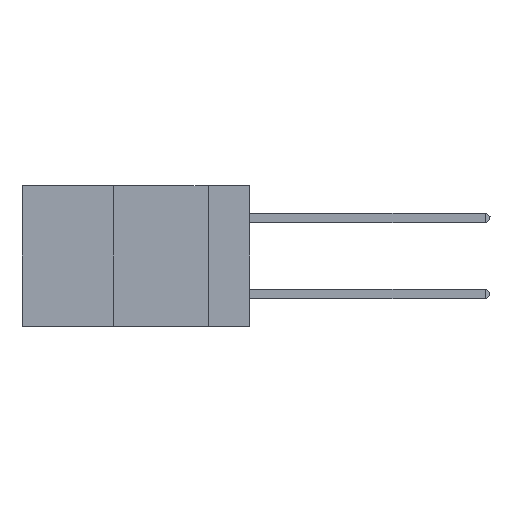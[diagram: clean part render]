
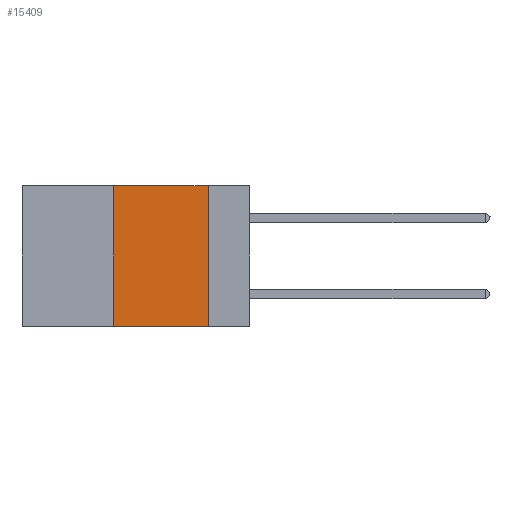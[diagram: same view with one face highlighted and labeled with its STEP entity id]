
A CAD part, left-side view. The second image highlights one B-rep face of the part: STEP entity #15409.
In plain terms, the highlighted planar face has unit normal (-1, 0, 0).
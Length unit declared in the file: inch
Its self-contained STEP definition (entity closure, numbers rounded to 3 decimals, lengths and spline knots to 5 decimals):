
#915 = LINE ( 'NONE', #6435, #17867 ) ;
#1359 = VERTEX_POINT ( 'NONE', #12019 ) ;
#1456 = CARTESIAN_POINT ( 'NONE',  ( 0., 0.11, -0.37 ) ) ;
#2284 = PLANE ( 'NONE',  #14364 ) ;
#3340 = VECTOR ( 'NONE', #15631, 39.37008 ) ;
#4250 = VERTEX_POINT ( 'NONE', #1456 ) ;
#5105 = LINE ( 'NONE', #9121, #7471 ) ;
#5170 = DIRECTION ( 'NONE',  ( 0., 0., -1. ) ) ;
#5252 = DIRECTION ( 'NONE',  ( 0., -1., 0. ) ) ;
#6081 = LINE ( 'NONE', #7360, #3340 ) ;
#6435 = CARTESIAN_POINT ( 'NONE',  ( 0., 0.6, 0. ) ) ;
#6571 = DIRECTION ( 'NONE',  ( 0., 0., -1. ) ) ;
#6595 = EDGE_CURVE ( 'NONE', #8617, #4250, #5105, .T. ) ;
#6596 = ORIENTED_EDGE ( 'NONE', *, *, #15986, .F. ) ;
#6624 = DIRECTION ( 'NONE',  ( 1., 0., 0. ) ) ;
#6927 = CARTESIAN_POINT ( 'NONE',  ( 0., 0.11, 0. ) ) ;
#7276 = ORIENTED_EDGE ( 'NONE', *, *, #15229, .F. ) ;
#7355 = ORIENTED_EDGE ( 'NONE', *, *, #6595, .T. ) ;
#7360 = CARTESIAN_POINT ( 'NONE',  ( 0., 0.36, 0. ) ) ;
#7471 = VECTOR ( 'NONE', #10667, 39.37008 ) ;
#8617 = VERTEX_POINT ( 'NONE', #13722 ) ;
#8921 = EDGE_CURVE ( 'NONE', #1359, #13538, #915, .T. ) ;
#9121 = CARTESIAN_POINT ( 'NONE',  ( 0., 0.6, -0.37 ) ) ;
#10021 = VECTOR ( 'NONE', #6571, 39.37008 ) ;
#10667 = DIRECTION ( 'NONE',  ( 0., -1., 0. ) ) ;
#12019 = CARTESIAN_POINT ( 'NONE',  ( 0., 0.36, 0. ) ) ;
#12246 = CARTESIAN_POINT ( 'NONE',  ( 0., 0.6, 0. ) ) ;
#12821 = EDGE_LOOP ( 'NONE', ( #6596, #14685, #7276, #7355 ) ) ;
#13538 = VERTEX_POINT ( 'NONE', #17346 ) ;
#13722 = CARTESIAN_POINT ( 'NONE',  ( 0., 0.36, -0.37 ) ) ;
#14364 = AXIS2_PLACEMENT_3D ( 'NONE', #12246, #6624, #5170 ) ;
#14685 = ORIENTED_EDGE ( 'NONE', *, *, #8921, .F. ) ;
#15229 = EDGE_CURVE ( 'NONE', #8617, #1359, #6081, .T. ) ;
#15409 = ADVANCED_FACE ( 'NONE', ( #16436 ), #2284, .F. ) ;
#15631 = DIRECTION ( 'NONE',  ( 0., 0., 1. ) ) ;
#15986 = EDGE_CURVE ( 'NONE', #13538, #4250, #17924, .T. ) ;
#16436 = FACE_OUTER_BOUND ( 'NONE', #12821, .T. ) ;
#17346 = CARTESIAN_POINT ( 'NONE',  ( 0., 0.11, 0. ) ) ;
#17867 = VECTOR ( 'NONE', #5252, 39.37008 ) ;
#17924 = LINE ( 'NONE', #6927, #10021 ) ;
